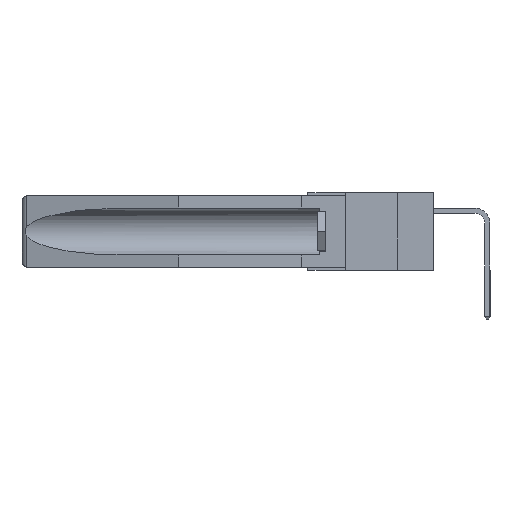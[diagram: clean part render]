
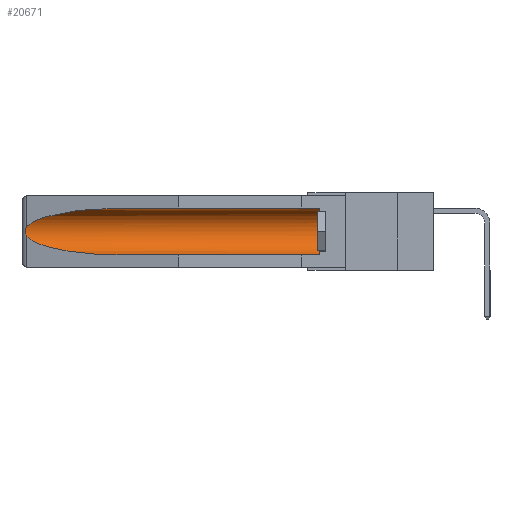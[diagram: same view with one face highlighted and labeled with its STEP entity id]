
A CAD part, left-side view. The second image highlights one B-rep face of the part: STEP entity #20671.
In plain terms, the highlighted cylindrical face has radius 2.857 mm (diameter 5.715 mm), a partial arc.
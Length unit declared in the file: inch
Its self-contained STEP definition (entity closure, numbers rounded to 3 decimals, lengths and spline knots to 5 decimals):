
#338 = B_SPLINE_CURVE_WITH_KNOTS ( 'NONE', 3,
 ( #21236, #17939, #667, #4130, #7372, #5912, #5608, #17626, #16114, #21089 ),
 .UNSPECIFIED., .F., .F.,
 ( 4, 2, 2, 2, 4 ),
 ( 0., 0.00029, 0.00058, 0.00087, 0.00117 ),
 .UNSPECIFIED. ) ;
#667 = CARTESIAN_POINT ( 'NONE',  ( 0.26654, 1.53092, -0.15636 ) ) ;
#819 = CARTESIAN_POINT ( 'NONE',  ( 0.25451, 1.48313, -0.24835 ) ) ;
#844 = CARTESIAN_POINT ( 'NONE',  ( 0.155, -0.30754, -0.284 ) ) ;
#1418 = CARTESIAN_POINT ( 'NONE',  ( 0.26537, 1.52718, -0.19328 ) ) ;
#1506 = VERTEX_POINT ( 'NONE', #21997 ) ;
#1636 = CIRCLE ( 'NONE', #7678, 0.1125 ) ;
#2117 = CARTESIAN_POINT ( 'NONE',  ( 0.155, 1.07973, -0.059 ) ) ;
#2498 = ORIENTED_EDGE ( 'NONE', *, *, #20876, .F. ) ;
#3283 = DIRECTION ( 'NONE',  ( 0., -1., 0. ) ) ;
#3440 = ORIENTED_EDGE ( 'NONE', *, *, #11864, .T. ) ;
#3824 = CARTESIAN_POINT ( 'NONE',  ( 0.26537, 1.52718, -0.14972 ) ) ;
#4130 = CARTESIAN_POINT ( 'NONE',  ( 0.2673, 1.5327, -0.16383 ) ) ;
#4781 = ORIENTED_EDGE ( 'NONE', *, *, #14763, .T. ) ;
#5608 = CARTESIAN_POINT ( 'NONE',  ( 0.2673, 1.53269, -0.17917 ) ) ;
#5912 = CARTESIAN_POINT ( 'NONE',  ( 0.2675, 1.53308, -0.17534 ) ) ;
#6906 = CYLINDRICAL_SURFACE ( 'NONE', #10814, 0.1125 ) ;
#7275 = ORIENTED_EDGE ( 'NONE', *, *, #20428, .T. ) ;
#7372 = CARTESIAN_POINT ( 'NONE',  ( 0.2675, 1.53308, -0.16763 ) ) ;
#7678 = AXIS2_PLACEMENT_3D ( 'NONE', #15181, #3283, #9963 ) ;
#7841 = ORIENTED_EDGE ( 'NONE', *, *, #17921, .T. ) ;
#8277 = FACE_OUTER_BOUND ( 'NONE', #13289, .T. ) ;
#8515 = VERTEX_POINT ( 'NONE', #19355 ) ;
#8987 = VECTOR ( 'NONE', #13606, 39.37008 ) ;
#9739 = CARTESIAN_POINT ( 'NONE',  ( 0.155, 1.07973, -0.059 ) ) ;
#9963 = DIRECTION ( 'NONE',  ( 0., 0., 1. ) ) ;
#10393 = DIRECTION ( 'NONE',  ( 0., 0., 1. ) ) ;
#10593 = CARTESIAN_POINT ( 'NONE',  ( 0.21114, 1.30732, -0.059 ) ) ;
#10814 = AXIS2_PLACEMENT_3D ( 'NONE', #15702, #12125, #10393 ) ;
#10922 = LINE ( 'NONE', #844, #14993 ) ;
#11841 = CARTESIAN_POINT ( 'NONE',  ( 0.26537, 1.52718, -0.14972 ) ) ;
#11864 = EDGE_CURVE ( 'NONE', #18198, #16244, #338, .T. ) ;
#12029 = EDGE_CURVE ( 'NONE', #16244, #1506, #14643, .T. ) ;
#12125 = DIRECTION ( 'NONE',  ( 0., 1., 0. ) ) ;
#12658 = VERTEX_POINT ( 'NONE', #9739 ) ;
#12936 = CARTESIAN_POINT ( 'NONE',  ( 0.21114, 1.30732, -0.284 ) ) ;
#13289 = EDGE_LOOP ( 'NONE', ( #7841, #3440, #17266, #2498, #7275, #4781 ) ) ;
#13606 = DIRECTION ( 'NONE',  ( 0., 1., 0. ) ) ;
#14087 = CARTESIAN_POINT ( 'NONE',  ( 0.25451, 1.48313, -0.09465 ) ) ;
#14643 =( BOUNDED_CURVE ( )  B_SPLINE_CURVE ( 3, ( #14747, #819, #12936, #18093 ),
 .UNSPECIFIED., .F., .F. ) 
 B_SPLINE_CURVE_WITH_KNOTS ( ( 4, 4 ),
 ( 0.1948, 1.5708 ),
 .UNSPECIFIED. ) 
 CURVE ( )  GEOMETRIC_REPRESENTATION_ITEM ( )  RATIONAL_B_SPLINE_CURVE ( ( 1., 0.848, 0.848, 1. ) ) 
 REPRESENTATION_ITEM ( '' )  );
#14747 = CARTESIAN_POINT ( 'NONE',  ( 0.26537, 1.52718, -0.19328 ) ) ;
#14763 = EDGE_CURVE ( 'NONE', #8515, #12658, #17634, .T. ) ;
#14993 = VECTOR ( 'NONE', #19624, 39.37008 ) ;
#15181 = CARTESIAN_POINT ( 'NONE',  ( 0.155, 0.126, -0.1715 ) ) ;
#15702 = CARTESIAN_POINT ( 'NONE',  ( 0.155, -0.30754, -0.1715 ) ) ;
#16114 = CARTESIAN_POINT ( 'NONE',  ( 0.26597, 1.5296, -0.19026 ) ) ;
#16244 = VERTEX_POINT ( 'NONE', #1418 ) ;
#17146 = CARTESIAN_POINT ( 'NONE',  ( 0.155, -0.30754, -0.059 ) ) ;
#17266 = ORIENTED_EDGE ( 'NONE', *, *, #12029, .T. ) ;
#17517 =( BOUNDED_CURVE ( )  B_SPLINE_CURVE ( 3, ( #2117, #10593, #14087, #3824 ),
 .UNSPECIFIED., .F., .F. ) 
 B_SPLINE_CURVE_WITH_KNOTS ( ( 4, 4 ),
 ( 4.71239, 6.08839 ),
 .UNSPECIFIED. ) 
 CURVE ( )  GEOMETRIC_REPRESENTATION_ITEM ( )  RATIONAL_B_SPLINE_CURVE ( ( 1., 0.848, 0.848, 1. ) ) 
 REPRESENTATION_ITEM ( '' )  );
#17626 = CARTESIAN_POINT ( 'NONE',  ( 0.26655, 1.53094, -0.18657 ) ) ;
#17634 = LINE ( 'NONE', #17146, #8987 ) ;
#17921 = EDGE_CURVE ( 'NONE', #12658, #18198, #17517, .T. ) ;
#17939 = CARTESIAN_POINT ( 'NONE',  ( 0.26597, 1.52961, -0.15275 ) ) ;
#17945 = VERTEX_POINT ( 'NONE', #19222 ) ;
#18093 = CARTESIAN_POINT ( 'NONE',  ( 0.155, 1.07973, -0.284 ) ) ;
#18198 = VERTEX_POINT ( 'NONE', #11841 ) ;
#19222 = CARTESIAN_POINT ( 'NONE',  ( 0.155, 0.126, -0.284 ) ) ;
#19355 = CARTESIAN_POINT ( 'NONE',  ( 0.155, 0.126, -0.059 ) ) ;
#19624 = DIRECTION ( 'NONE',  ( 0., 1., 0. ) ) ;
#20428 = EDGE_CURVE ( 'NONE', #17945, #8515, #1636, .T. ) ;
#20671 = ADVANCED_FACE ( 'NONE', ( #8277 ), #6906, .F. ) ;
#20876 = EDGE_CURVE ( 'NONE', #17945, #1506, #10922, .T. ) ;
#21089 = CARTESIAN_POINT ( 'NONE',  ( 0.26537, 1.52718, -0.19328 ) ) ;
#21236 = CARTESIAN_POINT ( 'NONE',  ( 0.26537, 1.52718, -0.14972 ) ) ;
#21997 = CARTESIAN_POINT ( 'NONE',  ( 0.155, 1.07973, -0.284 ) ) ;
